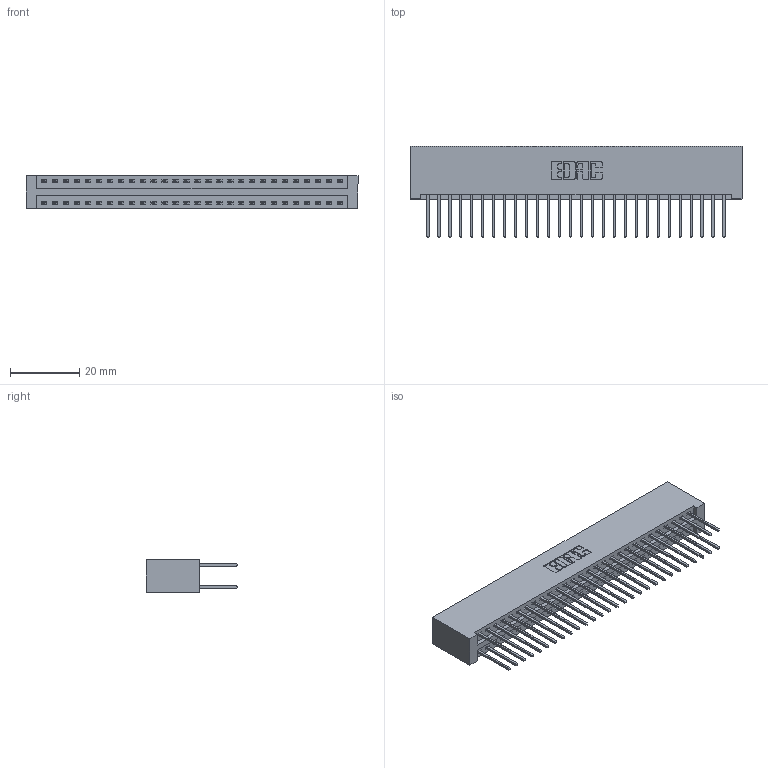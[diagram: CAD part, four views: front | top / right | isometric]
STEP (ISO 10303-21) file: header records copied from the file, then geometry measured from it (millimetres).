
FILE_DESCRIPTION (( 'STEP AP203' ), '1' );
FILE_NAME ('396-056-522-201.STEP', '2019-10-30T15:33:32', ( '' ), ( '' ), 'SwSTEP 2.0', 'SolidWorks 2016', '' );
FILE_SCHEMA (( 'CONFIG_CONTROL_DESIGN' ));
Length unit declared in the file: inch
Products named in the file (3): 345-292-001_345-293-122; 346 Part_No Mounting Lugs; 396-056-522-201
Assembly tree (57 placements, depth 2):
  396-056-522-201
    346 Part_No Mounting Lugs
    345-292-001_345-293-122  x56
Bounding box: 96.14 x 26.42 x 9.4 mm (x, y, z)
Volume: 9982.8 mm3; surface area: 14330.3 mm2
Topology: 57 solids, 57 shells, 3026 faces, 8985 edges, 5914 vertices
Faces by surface type: plane 2032, cylinder 994
Entity records: 19899 total; most frequent: CARTESIAN_POINT 3296, ORIENTED_EDGE 3230, DIRECTION 2951, EDGE_CURVE 1615, VECTOR 1379, LINE 1379, VERTEX_POINT 1074, AXIS2_PLACEMENT_3D 786
